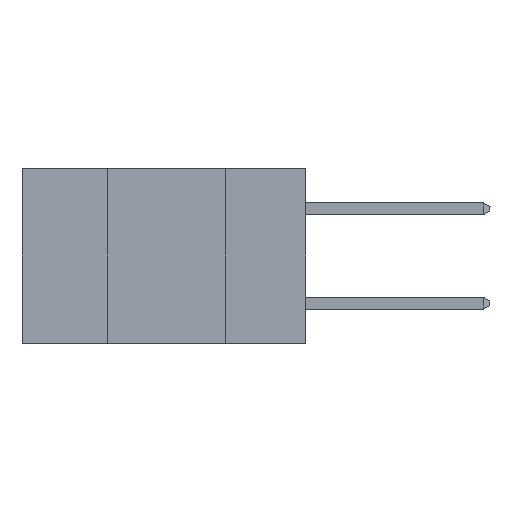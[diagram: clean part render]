
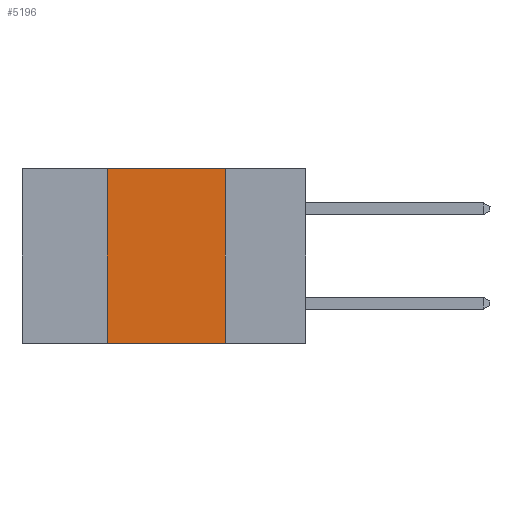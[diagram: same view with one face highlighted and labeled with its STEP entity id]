
A CAD part, left-side view. The second image highlights one B-rep face of the part: STEP entity #5196.
In plain terms, the highlighted planar face has unit normal (-1, 0, 0).
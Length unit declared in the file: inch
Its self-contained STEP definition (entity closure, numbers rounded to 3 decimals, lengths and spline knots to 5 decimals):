
#262 = DIRECTION ( 'NONE',  ( 0., 0., -1. ) ) ;
#1627 = EDGE_CURVE ( 'NONE', #22052, #15363, #22351, .T. ) ;
#1667 = VECTOR ( 'NONE', #12245, 39.37008 ) ;
#1986 = VECTOR ( 'NONE', #262, 39.37008 ) ;
#2417 = LINE ( 'NONE', #6621, #1986 ) ;
#2673 = ORIENTED_EDGE ( 'NONE', *, *, #1627, .F. ) ;
#3696 = CARTESIAN_POINT ( 'NONE',  ( 0., 0.42, 0. ) ) ;
#5196 = ADVANCED_FACE ( 'NONE', ( #16088 ), #6479, .F. ) ;
#5280 = EDGE_LOOP ( 'NONE', ( #15526, #10902, #2673, #12695 ) ) ;
#5730 = VECTOR ( 'NONE', #14439, 39.37008 ) ;
#6479 = PLANE ( 'NONE',  #22794 ) ;
#6621 = CARTESIAN_POINT ( 'NONE',  ( 0., 0.17, 0. ) ) ;
#7855 = CARTESIAN_POINT ( 'NONE',  ( 0., 0.42, 0. ) ) ;
#7901 = CARTESIAN_POINT ( 'NONE',  ( 0., 0.17, 0. ) ) ;
#10214 = LINE ( 'NONE', #12346, #20892 ) ;
#10902 = ORIENTED_EDGE ( 'NONE', *, *, #21376, .F. ) ;
#12245 = DIRECTION ( 'NONE',  ( 0., 0., 1. ) ) ;
#12346 = CARTESIAN_POINT ( 'NONE',  ( 0., 0.6, 0. ) ) ;
#12695 = ORIENTED_EDGE ( 'NONE', *, *, #24980, .T. ) ;
#14439 = DIRECTION ( 'NONE',  ( 0., -1., 0. ) ) ;
#15363 = VERTEX_POINT ( 'NONE', #7855 ) ;
#15381 = LINE ( 'NONE', #27301, #5730 ) ;
#15526 = ORIENTED_EDGE ( 'NONE', *, *, #20314, .F. ) ;
#16088 = FACE_OUTER_BOUND ( 'NONE', #5280, .T. ) ;
#17525 = CARTESIAN_POINT ( 'NONE',  ( 0., 0.17, -0.37 ) ) ;
#18703 = VERTEX_POINT ( 'NONE', #7901 ) ;
#20314 = EDGE_CURVE ( 'NONE', #18703, #25219, #2417, .T. ) ;
#20892 = VECTOR ( 'NONE', #27145, 39.37008 ) ;
#21361 = CARTESIAN_POINT ( 'NONE',  ( 0., 0.6, 0. ) ) ;
#21376 = EDGE_CURVE ( 'NONE', #15363, #18703, #10214, .T. ) ;
#22052 = VERTEX_POINT ( 'NONE', #23887 ) ;
#22351 = LINE ( 'NONE', #3696, #1667 ) ;
#22794 = AXIS2_PLACEMENT_3D ( 'NONE', #21361, #23472, #25628 ) ;
#23472 = DIRECTION ( 'NONE',  ( 1., 0., 0. ) ) ;
#23887 = CARTESIAN_POINT ( 'NONE',  ( 0., 0.42, -0.37 ) ) ;
#24980 = EDGE_CURVE ( 'NONE', #22052, #25219, #15381, .T. ) ;
#25219 = VERTEX_POINT ( 'NONE', #17525 ) ;
#25628 = DIRECTION ( 'NONE',  ( 0., 0., -1. ) ) ;
#27145 = DIRECTION ( 'NONE',  ( 0., -1., 0. ) ) ;
#27301 = CARTESIAN_POINT ( 'NONE',  ( 0., 0.6, -0.37 ) ) ;
